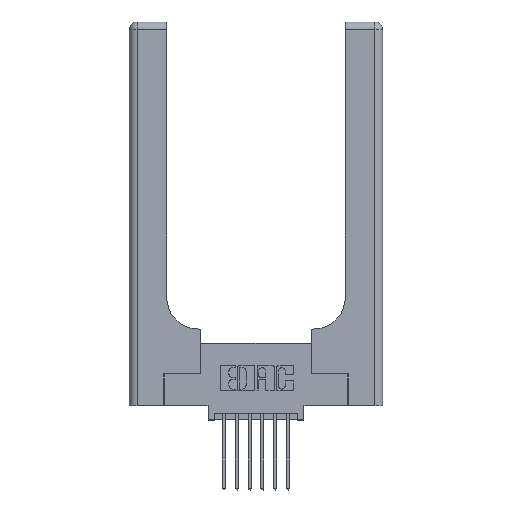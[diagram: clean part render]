
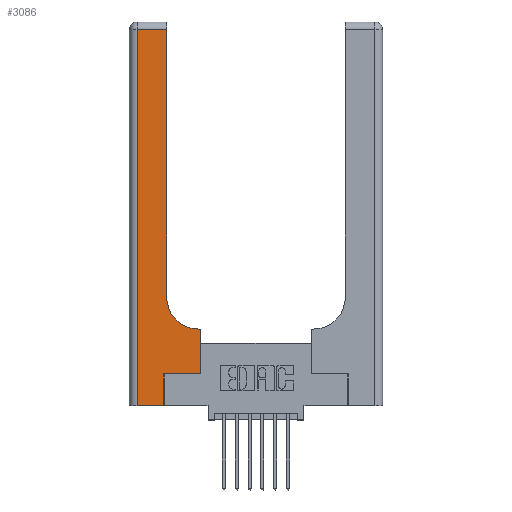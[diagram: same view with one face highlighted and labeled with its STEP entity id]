
A CAD part, top view. The second image highlights one B-rep face of the part: STEP entity #3086.
In plain terms, the highlighted planar face has unit normal (0, 0, 1).
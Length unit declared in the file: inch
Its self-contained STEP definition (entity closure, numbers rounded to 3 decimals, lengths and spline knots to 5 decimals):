
#98 = LINE ( 'NONE', #10728, #11971 ) ;
#519 = VECTOR ( 'NONE', #14832, 39.37008 ) ;
#586 = LINE ( 'NONE', #12315, #3306 ) ;
#624 = DIRECTION ( 'NONE',  ( 0., 0., -1. ) ) ;
#958 = VERTEX_POINT ( 'NONE', #3728 ) ;
#1159 = VERTEX_POINT ( 'NONE', #10504 ) ;
#1208 = ORIENTED_EDGE ( 'NONE', *, *, #9888, .T. ) ;
#1532 = VERTEX_POINT ( 'NONE', #12705 ) ;
#1539 = LINE ( 'NONE', #1806, #7629 ) ;
#1683 = CARTESIAN_POINT ( 'NONE',  ( 0.5585, 0.25, 0.37 ) ) ;
#1806 = CARTESIAN_POINT ( 'NONE',  ( 0.06, 3., 0.37 ) ) ;
#2728 = CARTESIAN_POINT ( 'NONE',  ( 0.5585, 0.25, 0.37 ) ) ;
#2801 = CARTESIAN_POINT ( 'NONE',  ( 0.5415, 0.6, 0.37 ) ) ;
#3086 = ADVANCED_FACE ( 'NONE', ( #3851 ), #11423, .F. ) ;
#3162 = LINE ( 'NONE', #6431, #12331 ) ;
#3306 = VECTOR ( 'NONE', #6535, 39.37008 ) ;
#3562 = VERTEX_POINT ( 'NONE', #6443 ) ;
#3728 = CARTESIAN_POINT ( 'NONE',  ( 0.06, 2.94, 0.37 ) ) ;
#3851 = FACE_OUTER_BOUND ( 'NONE', #8721, .T. ) ;
#3870 = DIRECTION ( 'NONE',  ( -1., 0., 0. ) ) ;
#3923 = VECTOR ( 'NONE', #13388, 39.37008 ) ;
#3986 = CARTESIAN_POINT ( 'NONE',  ( 0.2915, 0.85, 0.37 ) ) ;
#4015 = DIRECTION ( 'NONE',  ( 0., -1., 0. ) ) ;
#4228 = CARTESIAN_POINT ( 'NONE',  ( 0.06, 0., 0.37 ) ) ;
#4289 = ORIENTED_EDGE ( 'NONE', *, *, #12205, .T. ) ;
#4554 = CARTESIAN_POINT ( 'NONE',  ( 0., 3., 0.37 ) ) ;
#4621 = LINE ( 'NONE', #12230, #3923 ) ;
#5669 = DIRECTION ( 'NONE',  ( -1., 0., 0. ) ) ;
#6232 = LINE ( 'NONE', #12527, #519 ) ;
#6431 = CARTESIAN_POINT ( 'NONE',  ( 0.269, 0.25, 0.37 ) ) ;
#6443 = CARTESIAN_POINT ( 'NONE',  ( 0.5585, 0.6, 0.37 ) ) ;
#6461 = EDGE_CURVE ( 'NONE', #1159, #958, #6232, .T. ) ;
#6535 = DIRECTION ( 'NONE',  ( 1., 0., 0. ) ) ;
#6542 = LINE ( 'NONE', #8865, #11991 ) ;
#6834 = VERTEX_POINT ( 'NONE', #2801 ) ;
#6924 = ORIENTED_EDGE ( 'NONE', *, *, #9923, .T. ) ;
#6984 = VERTEX_POINT ( 'NONE', #4228 ) ;
#7464 = CARTESIAN_POINT ( 'NONE',  ( 0.5415, 0.85, 0.37 ) ) ;
#7481 = EDGE_CURVE ( 'NONE', #6834, #10910, #14533, .T. ) ;
#7485 = DIRECTION ( 'NONE',  ( 0., 1., 0. ) ) ;
#7593 = DIRECTION ( 'NONE',  ( 1., 0., 0. ) ) ;
#7629 = VECTOR ( 'NONE', #4015, 39.37008 ) ;
#7651 = ORIENTED_EDGE ( 'NONE', *, *, #10526, .T. ) ;
#7918 = AXIS2_PLACEMENT_3D ( 'NONE', #4554, #12594, #5669 ) ;
#8019 = ORIENTED_EDGE ( 'NONE', *, *, #14344, .T. ) ;
#8363 = ORIENTED_EDGE ( 'NONE', *, *, #7481, .T. ) ;
#8619 = DIRECTION ( 'NONE',  ( 1., 0., 0. ) ) ;
#8721 = EDGE_LOOP ( 'NONE', ( #6924, #13094, #1208, #4289, #10381, #7651, #8019, #14163, #8363 ) ) ;
#8865 = CARTESIAN_POINT ( 'NONE',  ( 0.269, 0., 0.37 ) ) ;
#9754 = EDGE_CURVE ( 'NONE', #3562, #6834, #98, .T. ) ;
#9888 = EDGE_CURVE ( 'NONE', #958, #6984, #1539, .T. ) ;
#9923 = EDGE_CURVE ( 'NONE', #10910, #1159, #4621, .T. ) ;
#9982 = DIRECTION ( 'NONE',  ( 0., 1., 0. ) ) ;
#10003 = EDGE_CURVE ( 'NONE', #1532, #10387, #6542, .T. ) ;
#10381 = ORIENTED_EDGE ( 'NONE', *, *, #10003, .T. ) ;
#10387 = VERTEX_POINT ( 'NONE', #10758 ) ;
#10504 = CARTESIAN_POINT ( 'NONE',  ( 0.2915, 2.94, 0.37 ) ) ;
#10526 = EDGE_CURVE ( 'NONE', #10387, #13587, #3162, .T. ) ;
#10728 = CARTESIAN_POINT ( 'NONE',  ( 0.2915, 0.6, 0.37 ) ) ;
#10758 = CARTESIAN_POINT ( 'NONE',  ( 0.269, 0.25, 0.37 ) ) ;
#10910 = VERTEX_POINT ( 'NONE', #3986 ) ;
#11423 = PLANE ( 'NONE',  #7918 ) ;
#11971 = VECTOR ( 'NONE', #3870, 39.37008 ) ;
#11991 = VECTOR ( 'NONE', #9982, 39.37008 ) ;
#12205 = EDGE_CURVE ( 'NONE', #6984, #1532, #586, .T. ) ;
#12230 = CARTESIAN_POINT ( 'NONE',  ( 0.2915, 3., 0.37 ) ) ;
#12315 = CARTESIAN_POINT ( 'NONE',  ( 0., 0., 0.37 ) ) ;
#12331 = VECTOR ( 'NONE', #7593, 39.37008 ) ;
#12527 = CARTESIAN_POINT ( 'NONE',  ( 0., 2.94, 0.37 ) ) ;
#12594 = DIRECTION ( 'NONE',  ( 0., 0., -1. ) ) ;
#12705 = CARTESIAN_POINT ( 'NONE',  ( 0.269, 0., 0.37 ) ) ;
#13094 = ORIENTED_EDGE ( 'NONE', *, *, #6461, .T. ) ;
#13388 = DIRECTION ( 'NONE',  ( 0., 1., 0. ) ) ;
#13560 = VECTOR ( 'NONE', #7485, 39.37008 ) ;
#13587 = VERTEX_POINT ( 'NONE', #2728 ) ;
#13912 = LINE ( 'NONE', #1683, #13560 ) ;
#14163 = ORIENTED_EDGE ( 'NONE', *, *, #9754, .T. ) ;
#14235 = AXIS2_PLACEMENT_3D ( 'NONE', #7464, #624, #8619 ) ;
#14344 = EDGE_CURVE ( 'NONE', #13587, #3562, #13912, .T. ) ;
#14533 = CIRCLE ( 'NONE', #14235, 0.25 ) ;
#14832 = DIRECTION ( 'NONE',  ( -1., 0., 0. ) ) ;
